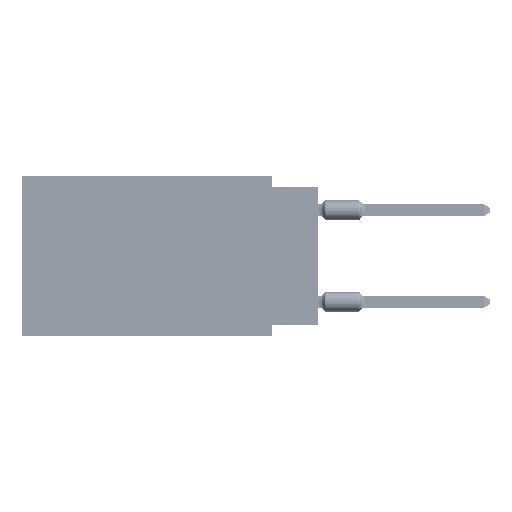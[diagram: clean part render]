
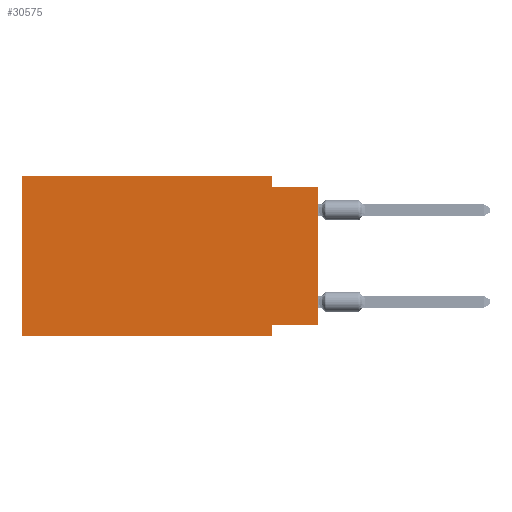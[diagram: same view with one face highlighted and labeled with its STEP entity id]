
A CAD part, left-side view. The second image highlights one B-rep face of the part: STEP entity #30575.
In plain terms, the highlighted planar face has unit normal (-1, 0, 0).
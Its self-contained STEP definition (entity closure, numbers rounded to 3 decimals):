
#786 = VECTOR ( 'NONE', #46135, 1000. ) ;
#1543 = FACE_OUTER_BOUND ( 'NONE', #48875, .T. ) ;
#5653 = LINE ( 'NONE', #17339, #8206 ) ;
#6270 = LINE ( 'NONE', #60335, #51825 ) ;
#8206 = VECTOR ( 'NONE', #65556, 1000. ) ;
#10811 = VERTEX_POINT ( 'NONE', #11888 ) ;
#11158 = LINE ( 'NONE', #76108, #38557 ) ;
#11201 = VERTEX_POINT ( 'NONE', #53785 ) ;
#11888 = CARTESIAN_POINT ( 'NONE',  ( 0., 16.383, -8.89 ) ) ;
#13475 = EDGE_CURVE ( 'NONE', #11201, #52832, #11158, .T. ) ;
#14889 = CARTESIAN_POINT ( 'NONE',  ( 0., 2.54, 0. ) ) ;
#17339 = CARTESIAN_POINT ( 'NONE',  ( 0., 0., 0. ) ) ;
#18614 = CARTESIAN_POINT ( 'NONE',  ( 0., 2.54, -8.255 ) ) ;
#18642 = EDGE_CURVE ( 'NONE', #10811, #59880, #61497, .T. ) ;
#19883 = VERTEX_POINT ( 'NONE', #62339 ) ;
#21468 = EDGE_CURVE ( 'NONE', #59880, #55866, #6270, .T. ) ;
#22081 = DIRECTION ( 'NONE',  ( 0., -1., 0. ) ) ;
#23227 = EDGE_CURVE ( 'NONE', #55866, #11201, #28766, .T. ) ;
#23292 = DIRECTION ( 'NONE',  ( 0., 0., -1. ) ) ;
#24105 = ORIENTED_EDGE ( 'NONE', *, *, #51045, .T. ) ;
#24379 = ORIENTED_EDGE ( 'NONE', *, *, #21468, .F. ) ;
#24923 = DIRECTION ( 'NONE',  ( 1., 0., 0. ) ) ;
#28766 = LINE ( 'NONE', #57926, #63205 ) ;
#29031 = CARTESIAN_POINT ( 'NONE',  ( 0., 16.383, -8.89 ) ) ;
#30575 = ADVANCED_FACE ( 'NONE', ( #1543 ), #55632, .F. ) ;
#32936 = EDGE_CURVE ( 'NONE', #68127, #66121, #35071, .T. ) ;
#32957 = LINE ( 'NONE', #33723, #786 ) ;
#33723 = CARTESIAN_POINT ( 'NONE',  ( 0., 0., -8.255 ) ) ;
#33888 = CARTESIAN_POINT ( 'NONE',  ( 0., 2.54, -8.89 ) ) ;
#35071 = LINE ( 'NONE', #41662, #73197 ) ;
#37733 = CARTESIAN_POINT ( 'NONE',  ( 0., 16.383, 0. ) ) ;
#38225 = CARTESIAN_POINT ( 'NONE',  ( 0., 0., -0.635 ) ) ;
#38557 = VECTOR ( 'NONE', #22081, 1000. ) ;
#39078 = DIRECTION ( 'NONE',  ( 0., 0., -1. ) ) ;
#39501 = ORIENTED_EDGE ( 'NONE', *, *, #32936, .F. ) ;
#40916 = AXIS2_PLACEMENT_3D ( 'NONE', #37733, #24923, #49020 ) ;
#41208 = EDGE_CURVE ( 'NONE', #10811, #66121, #45758, .T. ) ;
#41662 = CARTESIAN_POINT ( 'NONE',  ( 0., 2.54, -8.89 ) ) ;
#41992 = ORIENTED_EDGE ( 'NONE', *, *, #18642, .F. ) ;
#45758 = LINE ( 'NONE', #29031, #75852 ) ;
#46135 = DIRECTION ( 'NONE',  ( 0., 1., 0. ) ) ;
#47286 = DIRECTION ( 'NONE',  ( 0., -1., 0. ) ) ;
#48875 = EDGE_LOOP ( 'NONE', ( #24105, #70532, #74620, #24379, #41992, #65623, #39501, #69755 ) ) ;
#49020 = DIRECTION ( 'NONE',  ( 0., 0., -1. ) ) ;
#51045 = EDGE_CURVE ( 'NONE', #19883, #52832, #5653, .T. ) ;
#51825 = VECTOR ( 'NONE', #71992, 1000. ) ;
#52832 = VERTEX_POINT ( 'NONE', #38225 ) ;
#53408 = CARTESIAN_POINT ( 'NONE',  ( 0., 16.383, 0. ) ) ;
#53785 = CARTESIAN_POINT ( 'NONE',  ( 0., 2.54, -0.635 ) ) ;
#55632 = PLANE ( 'NONE',  #40916 ) ;
#55866 = VERTEX_POINT ( 'NONE', #14889 ) ;
#57926 = CARTESIAN_POINT ( 'NONE',  ( 0., 2.54, 0. ) ) ;
#59364 = EDGE_CURVE ( 'NONE', #19883, #68127, #32957, .T. ) ;
#59880 = VERTEX_POINT ( 'NONE', #53408 ) ;
#60335 = CARTESIAN_POINT ( 'NONE',  ( 0., 16.383, 0. ) ) ;
#61497 = LINE ( 'NONE', #74685, #73880 ) ;
#62266 = DIRECTION ( 'NONE',  ( 0., 0., 1. ) ) ;
#62339 = CARTESIAN_POINT ( 'NONE',  ( 0., 0., -8.255 ) ) ;
#63205 = VECTOR ( 'NONE', #23292, 1000. ) ;
#65556 = DIRECTION ( 'NONE',  ( 0., 0., 1. ) ) ;
#65623 = ORIENTED_EDGE ( 'NONE', *, *, #41208, .T. ) ;
#66121 = VERTEX_POINT ( 'NONE', #33888 ) ;
#68127 = VERTEX_POINT ( 'NONE', #18614 ) ;
#69755 = ORIENTED_EDGE ( 'NONE', *, *, #59364, .F. ) ;
#70532 = ORIENTED_EDGE ( 'NONE', *, *, #13475, .F. ) ;
#71992 = DIRECTION ( 'NONE',  ( 0., -1., 0. ) ) ;
#73197 = VECTOR ( 'NONE', #39078, 1000. ) ;
#73880 = VECTOR ( 'NONE', #62266, 1000. ) ;
#74620 = ORIENTED_EDGE ( 'NONE', *, *, #23227, .F. ) ;
#74685 = CARTESIAN_POINT ( 'NONE',  ( 0., 16.383, 0. ) ) ;
#75852 = VECTOR ( 'NONE', #47286, 1000. ) ;
#76108 = CARTESIAN_POINT ( 'NONE',  ( 0., 0., -0.635 ) ) ;
